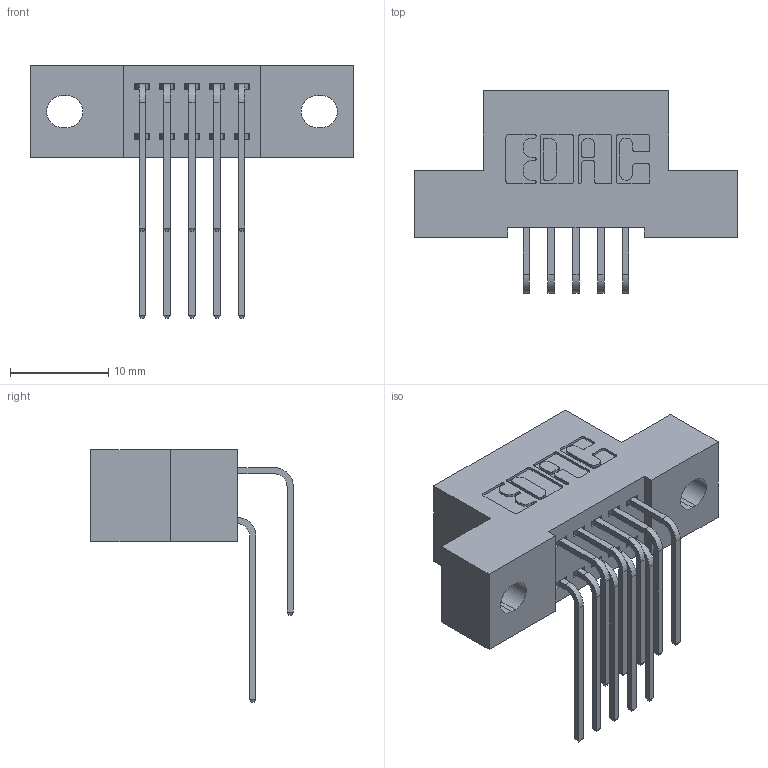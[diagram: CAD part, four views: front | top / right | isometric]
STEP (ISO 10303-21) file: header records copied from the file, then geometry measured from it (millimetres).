
FILE_DESCRIPTION (( 'STEP AP203' ), '1' );
FILE_NAME ('392-010-559-202.STEP', '2019-10-05T01:19:57', ( '' ), ( '' ), 'SwSTEP 2.0', 'SolidWorks 2016', '' );
FILE_SCHEMA (( 'CONFIG_CONTROL_DESIGN' ));
Length unit declared in the file: inch
Products named in the file (4): 342 Part_.128 Slot; 345-292-001_558 559 Tail - 1; 345-292-001_559 Tail - 2; 392-010-559-202
Assembly tree (11 placements, depth 2):
  392-010-559-202
    342 Part_.128 Slot
    345-292-001_558 559 Tail - 1  x5
    345-292-001_559 Tail - 2  x5
Bounding box: 33.02 x 20.64 x 25.78 mm (x, y, z)
Volume: 2797.3 mm3; surface area: 3662 mm2
Topology: 11 solids, 11 shells, 654 faces, 1921 edges, 1266 vertices
Faces by surface type: plane 450, cylinder 204
Entity records: 9789 total; most frequent: CARTESIAN_POINT 1717, ORIENTED_EDGE 1602, DIRECTION 1513, EDGE_CURVE 801, LINE 633, VECTOR 633, VERTEX_POINT 530, AXIS2_PLACEMENT_3D 440
